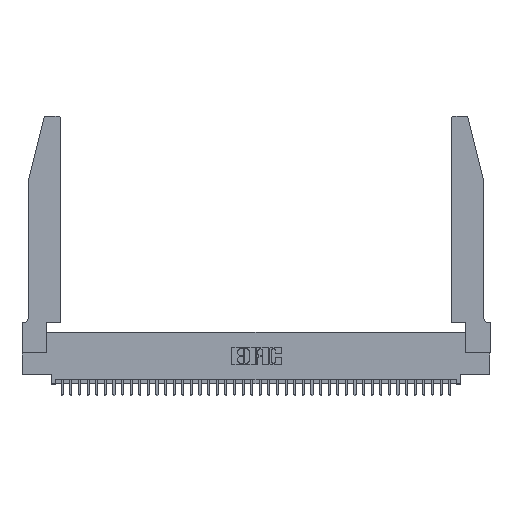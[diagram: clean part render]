
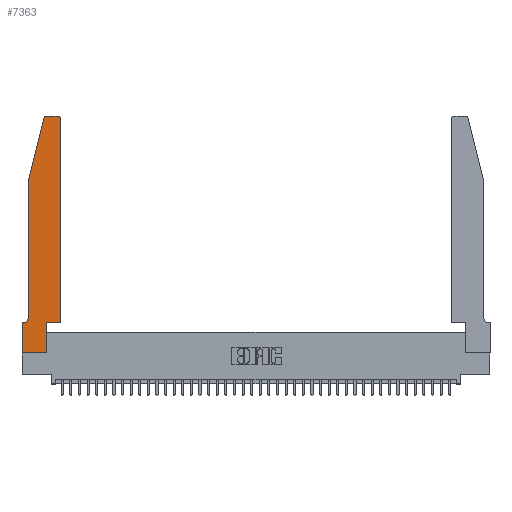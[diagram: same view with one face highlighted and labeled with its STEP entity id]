
A CAD part, top view. The second image highlights one B-rep face of the part: STEP entity #7363.
In plain terms, the highlighted planar face has unit normal (0, 0, 1).
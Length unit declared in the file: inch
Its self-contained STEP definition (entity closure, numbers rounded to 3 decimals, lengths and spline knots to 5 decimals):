
#713 = VERTEX_POINT ( 'NONE', #4994 ) ;
#927 = DIRECTION ( 'NONE',  ( 0., 1., 0. ) ) ;
#1011 = ORIENTED_EDGE ( 'NONE', *, *, #18238, .T. ) ;
#1526 = DIRECTION ( 'NONE',  ( 0., 0., 1. ) ) ;
#1608 = ORIENTED_EDGE ( 'NONE', *, *, #38277, .T. ) ;
#2038 = VERTEX_POINT ( 'NONE', #17108 ) ;
#2805 = DIRECTION ( 'NONE',  ( 0., -1., 0. ) ) ;
#2888 = CIRCLE ( 'NONE', #29620, 0.07 ) ;
#3623 = EDGE_CURVE ( 'NONE', #13657, #713, #38546, .T. ) ;
#4994 = CARTESIAN_POINT ( 'NONE',  ( 0., 0., 0.37 ) ) ;
#5418 = VERTEX_POINT ( 'NONE', #24182 ) ;
#6099 = CARTESIAN_POINT ( 'NONE',  ( 0., 0., 0.37 ) ) ;
#6807 = CARTESIAN_POINT ( 'NONE',  ( 0.2865, 0., 0.37 ) ) ;
#7179 = LINE ( 'NONE', #22246, #38514 ) ;
#7218 = VECTOR ( 'NONE', #2805, 39.37008 ) ;
#7337 = EDGE_CURVE ( 'NONE', #5418, #29855, #33888, .T. ) ;
#7363 = ADVANCED_FACE ( 'NONE', ( #16284 ), #38873, .T. ) ;
#7695 = CARTESIAN_POINT ( 'NONE',  ( 0.284, 2.72, 0.37 ) ) ;
#8118 = VERTEX_POINT ( 'NONE', #30832 ) ;
#8414 = CARTESIAN_POINT ( 'NONE',  ( 0.4205, 2.72, 0.37 ) ) ;
#8959 = LINE ( 'NONE', #6099, #16381 ) ;
#9440 = CARTESIAN_POINT ( 'NONE',  ( 0.0755, 2., 0.37 ) ) ;
#9727 = VERTEX_POINT ( 'NONE', #6807 ) ;
#10334 = VECTOR ( 'NONE', #14617, 39.37008 ) ;
#10866 = DIRECTION ( 'NONE',  ( 1., 0., 0. ) ) ;
#11432 = CARTESIAN_POINT ( 'NONE',  ( 0.2605, 2.75, 0.37 ) ) ;
#11602 = DIRECTION ( 'NONE',  ( 1., 0., 0. ) ) ;
#12032 = AXIS2_PLACEMENT_3D ( 'NONE', #8414, #30368, #11602 ) ;
#12073 = CARTESIAN_POINT ( 'NONE',  ( 0.25487, 2.72718, 0.37 ) ) ;
#12296 = DIRECTION ( 'NONE',  ( 1., 0., 0. ) ) ;
#12629 = DIRECTION ( 'NONE',  ( -0.239, -0.971, 0. ) ) ;
#13243 = LINE ( 'NONE', #9440, #37187 ) ;
#13603 = EDGE_CURVE ( 'NONE', #15133, #13657, #37135, .T. ) ;
#13657 = VERTEX_POINT ( 'NONE', #24049 ) ;
#13897 = EDGE_CURVE ( 'NONE', #14846, #25306, #7179, .T. ) ;
#14515 = VERTEX_POINT ( 'NONE', #16081 ) ;
#14617 = DIRECTION ( 'NONE',  ( -1., 0., 0. ) ) ;
#14846 = VERTEX_POINT ( 'NONE', #17713 ) ;
#15133 = VERTEX_POINT ( 'NONE', #34480 ) ;
#16081 = CARTESIAN_POINT ( 'NONE',  ( 0.4205, 2.75, 0.37 ) ) ;
#16144 = ORIENTED_EDGE ( 'NONE', *, *, #40029, .T. ) ;
#16259 = ORIENTED_EDGE ( 'NONE', *, *, #25158, .T. ) ;
#16284 = FACE_OUTER_BOUND ( 'NONE', #30812, .T. ) ;
#16367 = DIRECTION ( 'NONE',  ( 0., 0., -1. ) ) ;
#16381 = VECTOR ( 'NONE', #12296, 39.37008 ) ;
#16529 = VECTOR ( 'NONE', #927, 39.37008 ) ;
#16589 = CARTESIAN_POINT ( 'NONE',  ( 0.4505, 0.35, 0.37 ) ) ;
#17108 = CARTESIAN_POINT ( 'NONE',  ( 0.0755, 2., 0.37 ) ) ;
#17229 = CARTESIAN_POINT ( 'NONE',  ( 0., 0.35, 0.37 ) ) ;
#17296 = CARTESIAN_POINT ( 'NONE',  ( 0.4505, 2.72, 0.37 ) ) ;
#17457 = CARTESIAN_POINT ( 'NONE',  ( 0.0755, 0.42, 0.37 ) ) ;
#17713 = CARTESIAN_POINT ( 'NONE',  ( 0.4505, 0.35, 0.37 ) ) ;
#18238 = EDGE_CURVE ( 'NONE', #2038, #30866, #35084, .T. ) ;
#18678 = EDGE_CURVE ( 'NONE', #25306, #14515, #36986, .T. ) ;
#19618 = VECTOR ( 'NONE', #29199, 39.37008 ) ;
#20474 = CARTESIAN_POINT ( 'NONE',  ( 0.0755, 0.35, 0.37 ) ) ;
#21581 = LINE ( 'NONE', #16589, #19618 ) ;
#21704 = CARTESIAN_POINT ( 'NONE',  ( 0., 0., 0.37 ) ) ;
#21721 = ORIENTED_EDGE ( 'NONE', *, *, #35136, .T. ) ;
#21860 = AXIS2_PLACEMENT_3D ( 'NONE', #7695, #29659, #10866 ) ;
#22127 = EDGE_CURVE ( 'NONE', #29855, #2038, #13243, .T. ) ;
#22146 = CARTESIAN_POINT ( 'NONE',  ( 0.0755, 2., 0.37 ) ) ;
#22246 = CARTESIAN_POINT ( 'NONE',  ( 0.4505, 0.35, 0.37 ) ) ;
#23598 = ORIENTED_EDGE ( 'NONE', *, *, #22127, .T. ) ;
#23605 = DIRECTION ( 'NONE',  ( 1., 0., 0. ) ) ;
#24049 = CARTESIAN_POINT ( 'NONE',  ( 0., 0.35, 0.37 ) ) ;
#24182 = CARTESIAN_POINT ( 'NONE',  ( 0.284, 2.75, 0.37 ) ) ;
#25158 = EDGE_CURVE ( 'NONE', #9727, #8118, #33152, .T. ) ;
#25306 = VERTEX_POINT ( 'NONE', #17296 ) ;
#26838 = VECTOR ( 'NONE', #34489, 39.37008 ) ;
#26951 = VECTOR ( 'NONE', #39185, 39.37008 ) ;
#27543 = ORIENTED_EDGE ( 'NONE', *, *, #13897, .T. ) ;
#28115 = AXIS2_PLACEMENT_3D ( 'NONE', #17229, #1526, #23605 ) ;
#29199 = DIRECTION ( 'NONE',  ( 1., 0., 0. ) ) ;
#29415 = EDGE_CURVE ( 'NONE', #30866, #15133, #2888, .T. ) ;
#29620 = AXIS2_PLACEMENT_3D ( 'NONE', #35092, #16367, #38196 ) ;
#29659 = DIRECTION ( 'NONE',  ( 0., 0., 1. ) ) ;
#29855 = VERTEX_POINT ( 'NONE', #12073 ) ;
#30368 = DIRECTION ( 'NONE',  ( 0., 0., 1. ) ) ;
#30812 = EDGE_LOOP ( 'NONE', ( #1608, #35479, #23598, #1011, #30961, #32407, #36785, #21721, #16259, #16144, #27543, #31291 ) ) ;
#30832 = CARTESIAN_POINT ( 'NONE',  ( 0.2865, 0.35, 0.37 ) ) ;
#30866 = VERTEX_POINT ( 'NONE', #17457 ) ;
#30961 = ORIENTED_EDGE ( 'NONE', *, *, #29415, .T. ) ;
#31291 = ORIENTED_EDGE ( 'NONE', *, *, #18678, .T. ) ;
#32407 = ORIENTED_EDGE ( 'NONE', *, *, #13603, .T. ) ;
#33152 = LINE ( 'NONE', #38425, #16529 ) ;
#33888 = CIRCLE ( 'NONE', #21860, 0.03 ) ;
#34480 = CARTESIAN_POINT ( 'NONE',  ( 0.0055, 0.35, 0.37 ) ) ;
#34489 = DIRECTION ( 'NONE',  ( 0., -1., 0. ) ) ;
#35084 = LINE ( 'NONE', #22146, #26838 ) ;
#35092 = CARTESIAN_POINT ( 'NONE',  ( 0.0055, 0.42, 0.37 ) ) ;
#35136 = EDGE_CURVE ( 'NONE', #713, #9727, #8959, .T. ) ;
#35345 = LINE ( 'NONE', #11432, #10334 ) ;
#35479 = ORIENTED_EDGE ( 'NONE', *, *, #7337, .T. ) ;
#36785 = ORIENTED_EDGE ( 'NONE', *, *, #3623, .T. ) ;
#36986 = CIRCLE ( 'NONE', #12032, 0.03 ) ;
#37135 = LINE ( 'NONE', #20474, #26951 ) ;
#37187 = VECTOR ( 'NONE', #12629, 39.37008 ) ;
#37841 = DIRECTION ( 'NONE',  ( 0., 1., 0. ) ) ;
#38196 = DIRECTION ( 'NONE',  ( -1., 0., 0. ) ) ;
#38277 = EDGE_CURVE ( 'NONE', #14515, #5418, #35345, .T. ) ;
#38425 = CARTESIAN_POINT ( 'NONE',  ( 0.2865, 0.35, 0.37 ) ) ;
#38514 = VECTOR ( 'NONE', #37841, 39.37008 ) ;
#38546 = LINE ( 'NONE', #21704, #7218 ) ;
#38873 = PLANE ( 'NONE',  #28115 ) ;
#39185 = DIRECTION ( 'NONE',  ( -1., 0., 0. ) ) ;
#40029 = EDGE_CURVE ( 'NONE', #8118, #14846, #21581, .T. ) ;
